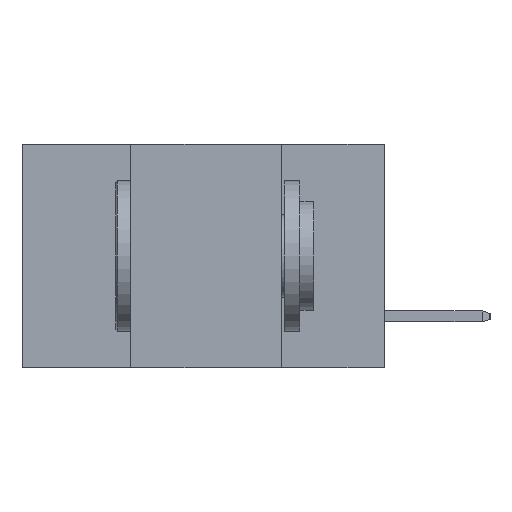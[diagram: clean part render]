
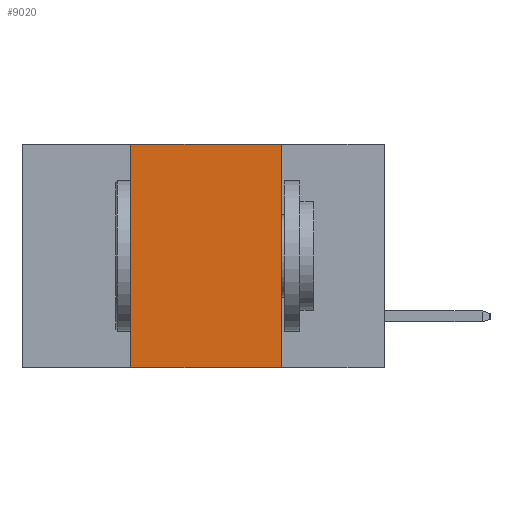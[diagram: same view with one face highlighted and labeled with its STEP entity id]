
A CAD part, left-side view. The second image highlights one B-rep face of the part: STEP entity #9020.
In plain terms, the highlighted planar face has unit normal (-1, 0, 0).
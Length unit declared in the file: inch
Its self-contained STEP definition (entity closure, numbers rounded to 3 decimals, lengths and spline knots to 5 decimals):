
#210 = CARTESIAN_POINT ( 'NONE',  ( 0., 0.6, 0. ) ) ;
#382 = VECTOR ( 'NONE', #6318, 39.37008 ) ;
#647 = LINE ( 'NONE', #6333, #7046 ) ;
#779 = EDGE_CURVE ( 'NONE', #7123, #7258, #647, .T. ) ;
#1128 = ORIENTED_EDGE ( 'NONE', *, *, #9891, .F. ) ;
#1859 = PLANE ( 'NONE',  #4557 ) ;
#2579 = LINE ( 'NONE', #6187, #382 ) ;
#2690 = VERTEX_POINT ( 'NONE', #4546 ) ;
#2698 = VERTEX_POINT ( 'NONE', #9103 ) ;
#2714 = DIRECTION ( 'NONE',  ( 0., 0., -1. ) ) ;
#4274 = DIRECTION ( 'NONE',  ( 0., 0., -1. ) ) ;
#4514 = DIRECTION ( 'NONE',  ( 0., -1., 0. ) ) ;
#4546 = CARTESIAN_POINT ( 'NONE',  ( 0., 0.42, -0.37 ) ) ;
#4557 = AXIS2_PLACEMENT_3D ( 'NONE', #210, #7431, #2714 ) ;
#4595 = VECTOR ( 'NONE', #5155, 39.37008 ) ;
#4744 = CARTESIAN_POINT ( 'NONE',  ( 0., 0.17, 0. ) ) ;
#4852 = EDGE_CURVE ( 'NONE', #2690, #7258, #2579, .T. ) ;
#5155 = DIRECTION ( 'NONE',  ( 0., 0., 1. ) ) ;
#5226 = ORIENTED_EDGE ( 'NONE', *, *, #779, .F. ) ;
#5467 = ORIENTED_EDGE ( 'NONE', *, *, #6908, .F. ) ;
#6187 = CARTESIAN_POINT ( 'NONE',  ( 0., 0.6, -0.37 ) ) ;
#6318 = DIRECTION ( 'NONE',  ( 0., -1., 0. ) ) ;
#6333 = CARTESIAN_POINT ( 'NONE',  ( 0., 0.17, -0.37 ) ) ;
#6626 = LINE ( 'NONE', #7414, #4595 ) ;
#6908 = EDGE_CURVE ( 'NONE', #2690, #2698, #6626, .T. ) ;
#7046 = VECTOR ( 'NONE', #4274, 39.37008 ) ;
#7123 = VERTEX_POINT ( 'NONE', #4744 ) ;
#7258 = VERTEX_POINT ( 'NONE', #9352 ) ;
#7414 = CARTESIAN_POINT ( 'NONE',  ( 0., 0.42, -0.37 ) ) ;
#7431 = DIRECTION ( 'NONE',  ( 1., 0., 0. ) ) ;
#7491 = ORIENTED_EDGE ( 'NONE', *, *, #4852, .T. ) ;
#7737 = EDGE_LOOP ( 'NONE', ( #5226, #1128, #5467, #7491 ) ) ;
#7976 = FACE_OUTER_BOUND ( 'NONE', #7737, .T. ) ;
#8687 = VECTOR ( 'NONE', #4514, 39.37008 ) ;
#9020 = ADVANCED_FACE ( 'NONE', ( #7976 ), #1859, .F. ) ;
#9103 = CARTESIAN_POINT ( 'NONE',  ( 0., 0.42, 0. ) ) ;
#9352 = CARTESIAN_POINT ( 'NONE',  ( 0., 0.17, -0.37 ) ) ;
#9780 = CARTESIAN_POINT ( 'NONE',  ( 0., 0.6, 0. ) ) ;
#9891 = EDGE_CURVE ( 'NONE', #2698, #7123, #10135, .T. ) ;
#10135 = LINE ( 'NONE', #9780, #8687 ) ;
